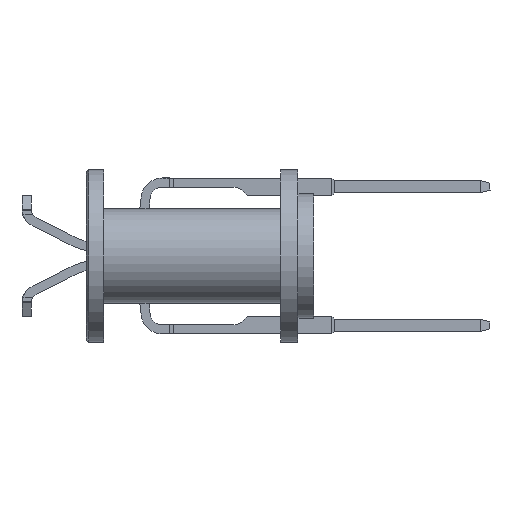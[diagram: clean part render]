
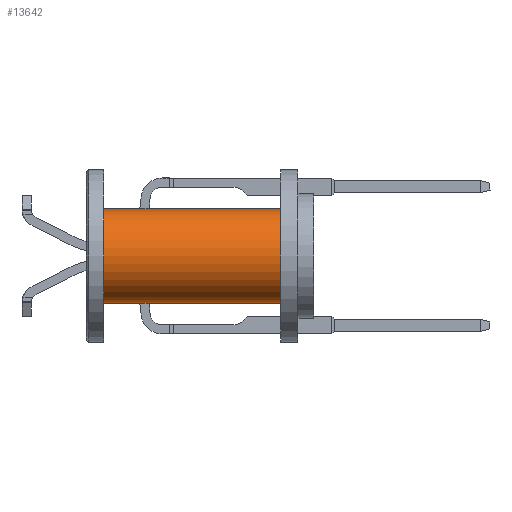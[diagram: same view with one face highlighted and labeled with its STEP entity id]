
A CAD part, left-side view. The second image highlights one B-rep face of the part: STEP entity #13642.
In plain terms, the highlighted cylindrical face has radius 1.727 mm (diameter 3.454 mm), a partial arc.
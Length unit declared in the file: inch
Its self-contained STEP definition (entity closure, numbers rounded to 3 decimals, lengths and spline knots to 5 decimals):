
#1058 = CARTESIAN_POINT ( 'NONE',  ( 0., 0.025, -0.068 ) ) ;
#1797 = DIRECTION ( 'NONE',  ( 0., 0., 1. ) ) ;
#2017 = VECTOR ( 'NONE', #18415, 39.37008 ) ;
#3840 = DIRECTION ( 'NONE',  ( 0., 0., -1. ) ) ;
#3956 = VECTOR ( 'NONE', #39772, 39.37008 ) ;
#4069 = CYLINDRICAL_SURFACE ( 'NONE', #32098, 0.068 ) ;
#8480 = CARTESIAN_POINT ( 'NONE',  ( 0., 0.328, 0.068 ) ) ;
#9741 = ORIENTED_EDGE ( 'NONE', *, *, #40669, .F. ) ;
#10453 = EDGE_LOOP ( 'NONE', ( #23774, #15625, #21471, #9741 ) ) ;
#10474 = EDGE_CURVE ( 'NONE', #18458, #40790, #37021, .T. ) ;
#10794 = EDGE_CURVE ( 'NONE', #18458, #20689, #43930, .T. ) ;
#13642 = ADVANCED_FACE ( 'NONE', ( #28525 ), #4069, .T. ) ;
#14687 = CARTESIAN_POINT ( 'NONE',  ( 0., 0.328, 0. ) ) ;
#15108 = AXIS2_PLACEMENT_3D ( 'NONE', #35266, #21664, #18199 ) ;
#15439 = CARTESIAN_POINT ( 'NONE',  ( 0., 0.28, 0. ) ) ;
#15625 = ORIENTED_EDGE ( 'NONE', *, *, #10794, .T. ) ;
#17179 = AXIS2_PLACEMENT_3D ( 'NONE', #15439, #29477, #1797 ) ;
#18199 = DIRECTION ( 'NONE',  ( 0., 0., 1. ) ) ;
#18415 = DIRECTION ( 'NONE',  ( 0., -1., 0. ) ) ;
#18458 = VERTEX_POINT ( 'NONE', #44326 ) ;
#19779 = CARTESIAN_POINT ( 'NONE',  ( 0., 0.28, -0.068 ) ) ;
#20689 = VERTEX_POINT ( 'NONE', #35547 ) ;
#21471 = ORIENTED_EDGE ( 'NONE', *, *, #36397, .T. ) ;
#21664 = DIRECTION ( 'NONE',  ( 0., 1., 0. ) ) ;
#23774 = ORIENTED_EDGE ( 'NONE', *, *, #10474, .F. ) ;
#25338 = LINE ( 'NONE', #26005, #2017 ) ;
#26005 = CARTESIAN_POINT ( 'NONE',  ( 0., 0.328, -0.068 ) ) ;
#28525 = FACE_OUTER_BOUND ( 'NONE', #10453, .T. ) ;
#29477 = DIRECTION ( 'NONE',  ( 0., 1., 0. ) ) ;
#30709 = DIRECTION ( 'NONE',  ( 0., -1., 0. ) ) ;
#31946 = VERTEX_POINT ( 'NONE', #1058 ) ;
#32098 = AXIS2_PLACEMENT_3D ( 'NONE', #14687, #30709, #3840 ) ;
#34239 = CIRCLE ( 'NONE', #15108, 0.068 ) ;
#35266 = CARTESIAN_POINT ( 'NONE',  ( 0., 0.025, 0. ) ) ;
#35547 = CARTESIAN_POINT ( 'NONE',  ( 0., 0.025, 0.068 ) ) ;
#36397 = EDGE_CURVE ( 'NONE', #20689, #31946, #34239, .T. ) ;
#37021 = CIRCLE ( 'NONE', #17179, 0.068 ) ;
#39772 = DIRECTION ( 'NONE',  ( 0., -1., 0. ) ) ;
#40669 = EDGE_CURVE ( 'NONE', #40790, #31946, #25338, .T. ) ;
#40790 = VERTEX_POINT ( 'NONE', #19779 ) ;
#43930 = LINE ( 'NONE', #8480, #3956 ) ;
#44326 = CARTESIAN_POINT ( 'NONE',  ( 0., 0.28, 0.068 ) ) ;
